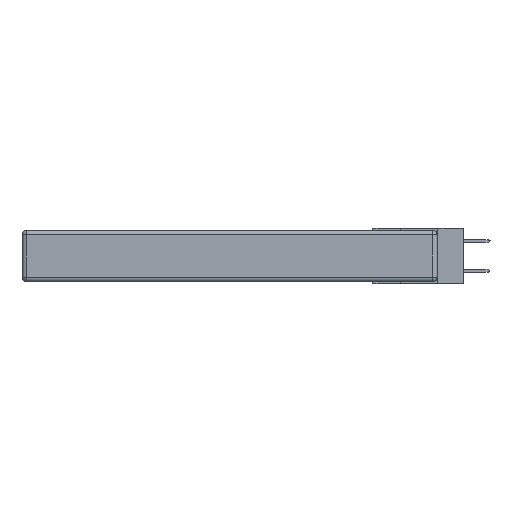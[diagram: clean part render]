
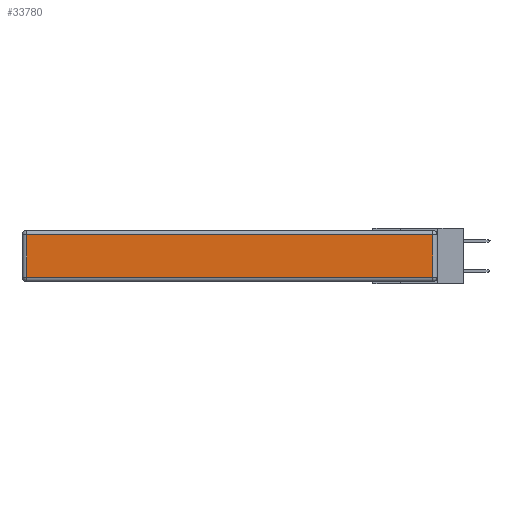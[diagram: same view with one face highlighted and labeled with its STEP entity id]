
A CAD part, left-side view. The second image highlights one B-rep face of the part: STEP entity #33780.
In plain terms, the highlighted planar face has unit normal (-1, 0, 0).
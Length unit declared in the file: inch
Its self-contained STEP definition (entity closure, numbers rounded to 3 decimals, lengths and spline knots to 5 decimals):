
#1437 = LINE ( 'NONE', #22797, #9758 ) ;
#1790 = CARTESIAN_POINT ( 'NONE',  ( 0., 0., -0.313 ) ) ;
#2435 = VERTEX_POINT ( 'NONE', #8864 ) ;
#3813 = AXIS2_PLACEMENT_3D ( 'NONE', #9086, #27317, #27204 ) ;
#4150 = VECTOR ( 'NONE', #25768, 39.37008 ) ;
#7611 = ORIENTED_EDGE ( 'NONE', *, *, #30645, .T. ) ;
#8864 = CARTESIAN_POINT ( 'NONE',  ( 0., 0.03, -0.03 ) ) ;
#9086 = CARTESIAN_POINT ( 'NONE',  ( 0., 0., -0.343 ) ) ;
#9642 = CARTESIAN_POINT ( 'NONE',  ( 0., 2.72, -0.03 ) ) ;
#9758 = VECTOR ( 'NONE', #25482, 39.37008 ) ;
#10467 = VERTEX_POINT ( 'NONE', #12489 ) ;
#10955 = CARTESIAN_POINT ( 'NONE',  ( 0., 0.03, -0.313 ) ) ;
#11214 = LINE ( 'NONE', #15370, #4150 ) ;
#12489 = CARTESIAN_POINT ( 'NONE',  ( 0., 2.72, -0.313 ) ) ;
#12803 = ORIENTED_EDGE ( 'NONE', *, *, #27060, .T. ) ;
#13853 = LINE ( 'NONE', #1790, #14298 ) ;
#14298 = VECTOR ( 'NONE', #26500, 39.37008 ) ;
#15370 = CARTESIAN_POINT ( 'NONE',  ( 0., 0.03, -0.343 ) ) ;
#15715 = FACE_OUTER_BOUND ( 'NONE', #28329, .T. ) ;
#16566 = VECTOR ( 'NONE', #30649, 39.37008 ) ;
#16900 = PLANE ( 'NONE',  #3813 ) ;
#19010 = VERTEX_POINT ( 'NONE', #9642 ) ;
#19827 = ORIENTED_EDGE ( 'NONE', *, *, #30582, .T. ) ;
#20232 = CARTESIAN_POINT ( 'NONE',  ( 0., 2.72, -0.343 ) ) ;
#21360 = VERTEX_POINT ( 'NONE', #10955 ) ;
#22797 = CARTESIAN_POINT ( 'NONE',  ( 0., 2.75, -0.03 ) ) ;
#24936 = ORIENTED_EDGE ( 'NONE', *, *, #33982, .T. ) ;
#25482 = DIRECTION ( 'NONE',  ( 0., 1., 0. ) ) ;
#25642 = LINE ( 'NONE', #20232, #16566 ) ;
#25768 = DIRECTION ( 'NONE',  ( 0., 0., 1. ) ) ;
#26500 = DIRECTION ( 'NONE',  ( 0., -1., 0. ) ) ;
#27060 = EDGE_CURVE ( 'NONE', #19010, #10467, #25642, .T. ) ;
#27204 = DIRECTION ( 'NONE',  ( 0., 0., 1. ) ) ;
#27317 = DIRECTION ( 'NONE',  ( -1., 0., 0. ) ) ;
#28329 = EDGE_LOOP ( 'NONE', ( #7611, #24936, #19827, #12803 ) ) ;
#30582 = EDGE_CURVE ( 'NONE', #2435, #19010, #1437, .T. ) ;
#30645 = EDGE_CURVE ( 'NONE', #10467, #21360, #13853, .T. ) ;
#30649 = DIRECTION ( 'NONE',  ( 0., 0., -1. ) ) ;
#33780 = ADVANCED_FACE ( 'NONE', ( #15715 ), #16900, .T. ) ;
#33982 = EDGE_CURVE ( 'NONE', #21360, #2435, #11214, .T. ) ;
